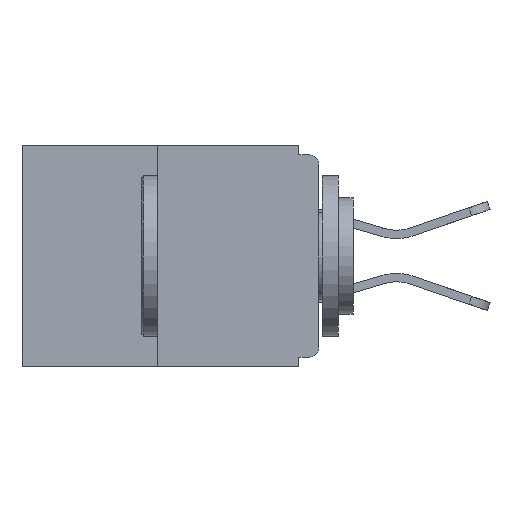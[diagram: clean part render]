
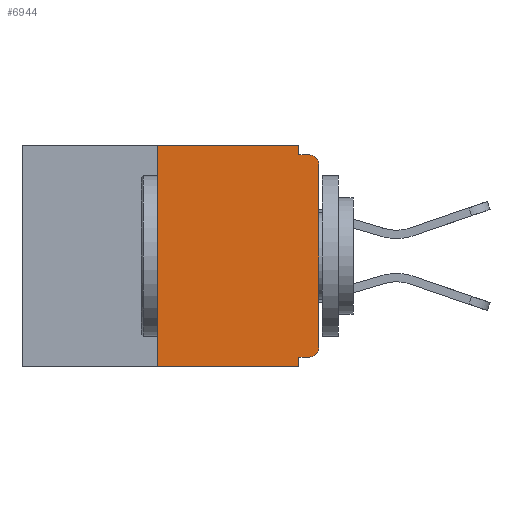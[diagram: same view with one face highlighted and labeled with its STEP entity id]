
A CAD part, left-side view. The second image highlights one B-rep face of the part: STEP entity #6944.
In plain terms, the highlighted planar face has unit normal (-1, 0, 0).
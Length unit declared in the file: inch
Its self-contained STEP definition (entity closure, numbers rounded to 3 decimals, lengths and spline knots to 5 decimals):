
#426 = DIRECTION ( 'NONE',  ( 0., 0., 1. ) ) ;
#550 = ORIENTED_EDGE ( 'NONE', *, *, #2342, .F. ) ;
#1717 = EDGE_CURVE ( 'NONE', #15795, #11851, #11897, .T. ) ;
#1923 = ORIENTED_EDGE ( 'NONE', *, *, #1717, .T. ) ;
#2342 = EDGE_CURVE ( 'NONE', #15425, #11851, #15205, .T. ) ;
#2575 = LINE ( 'NONE', #8459, #22088 ) ;
#2722 = CARTESIAN_POINT ( 'NONE',  ( 0., 0.015, -0.313 ) ) ;
#2757 = CARTESIAN_POINT ( 'NONE',  ( 0., 0.015, -0.015 ) ) ;
#2767 = ORIENTED_EDGE ( 'NONE', *, *, #3998, .F. ) ;
#3110 = DIRECTION ( 'NONE',  ( 0., 0., -1. ) ) ;
#3188 = EDGE_CURVE ( 'NONE', #6882, #15795, #16271, .T. ) ;
#3843 = ORIENTED_EDGE ( 'NONE', *, *, #3188, .T. ) ;
#3998 = EDGE_CURVE ( 'NONE', #11999, #15425, #2575, .T. ) ;
#4355 = VECTOR ( 'NONE', #19574, 39.37008 ) ;
#4978 = CARTESIAN_POINT ( 'NONE',  ( 0., 0.031, -0.343 ) ) ;
#5111 = ORIENTED_EDGE ( 'NONE', *, *, #11033, .F. ) ;
#5151 = CARTESIAN_POINT ( 'NONE',  ( 0., 0.46, 0. ) ) ;
#5548 = LINE ( 'NONE', #4978, #19761 ) ;
#6631 = LINE ( 'NONE', #21007, #20271 ) ;
#6689 = VERTEX_POINT ( 'NONE', #10028 ) ;
#6882 = VERTEX_POINT ( 'NONE', #21345 ) ;
#6944 = ADVANCED_FACE ( 'NONE', ( #13101 ), #7117, .F. ) ;
#7050 = VERTEX_POINT ( 'NONE', #21885 ) ;
#7093 = VECTOR ( 'NONE', #20403, 39.37008 ) ;
#7117 = PLANE ( 'NONE',  #13131 ) ;
#7226 = DIRECTION ( 'NONE',  ( 0., 0., 1. ) ) ;
#8117 = EDGE_CURVE ( 'NONE', #8506, #11491, #6631, .T. ) ;
#8459 = CARTESIAN_POINT ( 'NONE',  ( 0., 0.031, 0. ) ) ;
#8506 = VERTEX_POINT ( 'NONE', #22117 ) ;
#9196 = ORIENTED_EDGE ( 'NONE', *, *, #22499, .F. ) ;
#9578 = CARTESIAN_POINT ( 'NONE',  ( 0., 0., -0.328 ) ) ;
#9796 = ORIENTED_EDGE ( 'NONE', *, *, #17668, .T. ) ;
#10028 = CARTESIAN_POINT ( 'NONE',  ( 0., 0.031, -0.328 ) ) ;
#10321 = EDGE_LOOP ( 'NONE', ( #15927, #20306, #21711, #9196, #5111, #9796, #3843, #1923, #550, #2767 ) ) ;
#10772 = CARTESIAN_POINT ( 'NONE',  ( 0., 0.031, 0. ) ) ;
#10974 = EDGE_CURVE ( 'NONE', #8506, #7050, #13220, .T. ) ;
#11033 = EDGE_CURVE ( 'NONE', #20372, #6689, #11815, .T. ) ;
#11491 = VERTEX_POINT ( 'NONE', #13010 ) ;
#11815 = LINE ( 'NONE', #9578, #7093 ) ;
#11851 = VERTEX_POINT ( 'NONE', #2757 ) ;
#11897 = CIRCLE ( 'NONE', #18679, 0.015 ) ;
#11968 = DIRECTION ( 'NONE',  ( 0., 0., -1. ) ) ;
#11999 = VERTEX_POINT ( 'NONE', #10772 ) ;
#12006 = DIRECTION ( 'NONE',  ( -1., 0., 0. ) ) ;
#12084 = CARTESIAN_POINT ( 'NONE',  ( 0., 0.015, -0.03 ) ) ;
#12158 = DIRECTION ( 'NONE',  ( 0., 0., -1. ) ) ;
#12375 = CARTESIAN_POINT ( 'NONE',  ( 0., 0., 0. ) ) ;
#12395 = VECTOR ( 'NONE', #7226, 39.37008 ) ;
#12940 = DIRECTION ( 'NONE',  ( 0., -1., 0. ) ) ;
#13010 = CARTESIAN_POINT ( 'NONE',  ( 0., 0.031, -0.343 ) ) ;
#13101 = FACE_OUTER_BOUND ( 'NONE', #10321, .T. ) ;
#13113 = CARTESIAN_POINT ( 'NONE',  ( 0., 0.25, 0. ) ) ;
#13131 = AXIS2_PLACEMENT_3D ( 'NONE', #14267, #15992, #16059 ) ;
#13220 = LINE ( 'NONE', #13113, #20169 ) ;
#13677 = CARTESIAN_POINT ( 'NONE',  ( 0., 0., -0.03 ) ) ;
#14267 = CARTESIAN_POINT ( 'NONE',  ( 0., 0.46, 0. ) ) ;
#14840 = CARTESIAN_POINT ( 'NONE',  ( 0., 0.015, -0.328 ) ) ;
#15205 = LINE ( 'NONE', #17964, #15471 ) ;
#15425 = VERTEX_POINT ( 'NONE', #22493 ) ;
#15471 = VECTOR ( 'NONE', #12940, 39.37008 ) ;
#15795 = VERTEX_POINT ( 'NONE', #13677 ) ;
#15800 = DIRECTION ( 'NONE',  ( 0., -1., 0. ) ) ;
#15927 = ORIENTED_EDGE ( 'NONE', *, *, #17855, .F. ) ;
#15992 = DIRECTION ( 'NONE',  ( 1., 0., 0. ) ) ;
#16059 = DIRECTION ( 'NONE',  ( 0., 0., -1. ) ) ;
#16271 = LINE ( 'NONE', #12375, #12395 ) ;
#17069 = DIRECTION ( 'NONE',  ( -1., 0., 0. ) ) ;
#17668 = EDGE_CURVE ( 'NONE', #20372, #6882, #19736, .T. ) ;
#17855 = EDGE_CURVE ( 'NONE', #7050, #11999, #20238, .T. ) ;
#17964 = CARTESIAN_POINT ( 'NONE',  ( 0., 0., -0.015 ) ) ;
#18270 = AXIS2_PLACEMENT_3D ( 'NONE', #2722, #17069, #18701 ) ;
#18679 = AXIS2_PLACEMENT_3D ( 'NONE', #12084, #12006, #3110 ) ;
#18701 = DIRECTION ( 'NONE',  ( 0., 0., -1. ) ) ;
#19574 = DIRECTION ( 'NONE',  ( 0., -1., 0. ) ) ;
#19736 = CIRCLE ( 'NONE', #18270, 0.015 ) ;
#19761 = VECTOR ( 'NONE', #12158, 39.37008 ) ;
#20169 = VECTOR ( 'NONE', #426, 39.37008 ) ;
#20238 = LINE ( 'NONE', #5151, #4355 ) ;
#20271 = VECTOR ( 'NONE', #15800, 39.37008 ) ;
#20306 = ORIENTED_EDGE ( 'NONE', *, *, #10974, .F. ) ;
#20372 = VERTEX_POINT ( 'NONE', #14840 ) ;
#20403 = DIRECTION ( 'NONE',  ( 0., 1., 0. ) ) ;
#21007 = CARTESIAN_POINT ( 'NONE',  ( 0., 0.46, -0.343 ) ) ;
#21345 = CARTESIAN_POINT ( 'NONE',  ( 0., 0., -0.313 ) ) ;
#21711 = ORIENTED_EDGE ( 'NONE', *, *, #8117, .T. ) ;
#21885 = CARTESIAN_POINT ( 'NONE',  ( 0., 0.25, 0. ) ) ;
#22088 = VECTOR ( 'NONE', #11968, 39.37008 ) ;
#22117 = CARTESIAN_POINT ( 'NONE',  ( 0., 0.25, -0.343 ) ) ;
#22493 = CARTESIAN_POINT ( 'NONE',  ( 0., 0.031, -0.015 ) ) ;
#22499 = EDGE_CURVE ( 'NONE', #6689, #11491, #5548, .T. ) ;
